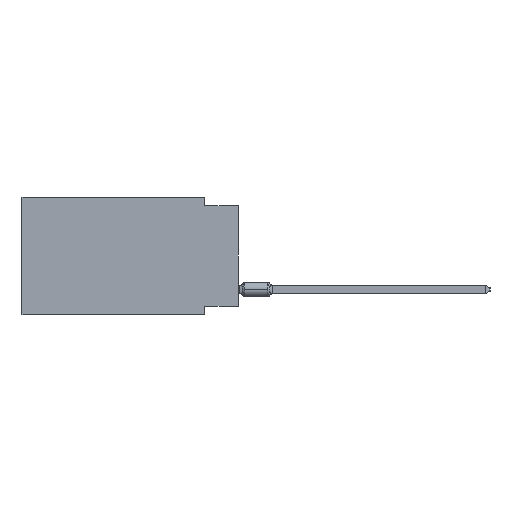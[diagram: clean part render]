
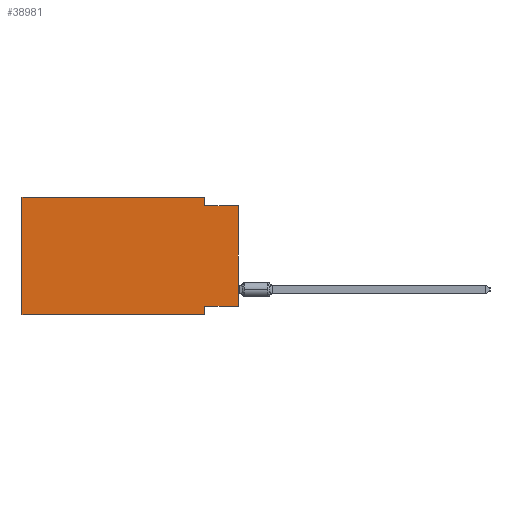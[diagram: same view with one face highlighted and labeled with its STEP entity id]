
A CAD part, left-side view. The second image highlights one B-rep face of the part: STEP entity #38981.
In plain terms, the highlighted planar face has unit normal (-1, 0, 0).
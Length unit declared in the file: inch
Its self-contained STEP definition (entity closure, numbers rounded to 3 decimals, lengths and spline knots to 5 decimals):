
#219 = VECTOR ( 'NONE', #7970, 39.37008 ) ;
#351 = DIRECTION ( 'NONE',  ( 0., 0., 1. ) ) ;
#927 = CARTESIAN_POINT ( 'NONE',  ( 0., 0.1, -0.325 ) ) ;
#3507 = ORIENTED_EDGE ( 'NONE', *, *, #48282, .F. ) ;
#4763 = CARTESIAN_POINT ( 'NONE',  ( 0., 0., -0.025 ) ) ;
#4801 = VERTEX_POINT ( 'NONE', #927 ) ;
#5118 = DIRECTION ( 'NONE',  ( 1., 0., 0. ) ) ;
#5246 = EDGE_CURVE ( 'NONE', #30728, #7656, #63425, .T. ) ;
#6955 = CARTESIAN_POINT ( 'NONE',  ( 0., 0.1, -0.35 ) ) ;
#7656 = VERTEX_POINT ( 'NONE', #24314 ) ;
#7919 = CARTESIAN_POINT ( 'NONE',  ( 0., 0., 0. ) ) ;
#7970 = DIRECTION ( 'NONE',  ( 0., -1., 0. ) ) ;
#8105 = EDGE_CURVE ( 'NONE', #7656, #64206, #9751, .T. ) ;
#8794 = DIRECTION ( 'NONE',  ( 0., -1., 0. ) ) ;
#9710 = LINE ( 'NONE', #46123, #57536 ) ;
#9751 = LINE ( 'NONE', #65556, #13404 ) ;
#10563 = VERTEX_POINT ( 'NONE', #36013 ) ;
#12307 = DIRECTION ( 'NONE',  ( 0., 0., -1. ) ) ;
#12536 = LINE ( 'NONE', #26581, #15799 ) ;
#13404 = VECTOR ( 'NONE', #19788, 39.37008 ) ;
#14592 = ORIENTED_EDGE ( 'NONE', *, *, #45447, .F. ) ;
#15783 = LINE ( 'NONE', #4763, #37073 ) ;
#15799 = VECTOR ( 'NONE', #57007, 39.37008 ) ;
#16535 = VERTEX_POINT ( 'NONE', #58576 ) ;
#16675 = LINE ( 'NONE', #6955, #18326 ) ;
#18326 = VECTOR ( 'NONE', #12307, 39.37008 ) ;
#19788 = DIRECTION ( 'NONE',  ( 0., 0., -1. ) ) ;
#20963 = ORIENTED_EDGE ( 'NONE', *, *, #8105, .F. ) ;
#22173 = VECTOR ( 'NONE', #58391, 39.37008 ) ;
#23159 = CARTESIAN_POINT ( 'NONE',  ( 0., 0.645, -0.35 ) ) ;
#24314 = CARTESIAN_POINT ( 'NONE',  ( 0., 0.1, 0. ) ) ;
#25510 = PLANE ( 'NONE',  #46611 ) ;
#25827 = FACE_OUTER_BOUND ( 'NONE', #31865, .T. ) ;
#25960 = CARTESIAN_POINT ( 'NONE',  ( 0., 0.1, -0.025 ) ) ;
#26371 = ORIENTED_EDGE ( 'NONE', *, *, #64893, .T. ) ;
#26581 = CARTESIAN_POINT ( 'NONE',  ( 0., 0., -0.325 ) ) ;
#28676 = EDGE_CURVE ( 'NONE', #16535, #61538, #53703, .T. ) ;
#30728 = VERTEX_POINT ( 'NONE', #41770 ) ;
#31443 = DIRECTION ( 'NONE',  ( 0., -1., 0. ) ) ;
#31865 = EDGE_LOOP ( 'NONE', ( #55086, #3507, #20963, #49716, #14592, #26371, #48968, #47297 ) ) ;
#32692 = CARTESIAN_POINT ( 'NONE',  ( 0., 0.645, 0. ) ) ;
#36013 = CARTESIAN_POINT ( 'NONE',  ( 0., 0.645, -0.35 ) ) ;
#37073 = VECTOR ( 'NONE', #31443, 39.37008 ) ;
#37854 = LINE ( 'NONE', #23159, #42801 ) ;
#38981 = ADVANCED_FACE ( 'NONE', ( #25827 ), #25510, .F. ) ;
#39543 = CARTESIAN_POINT ( 'NONE',  ( 0., 0.1, -0.35 ) ) ;
#40150 = VERTEX_POINT ( 'NONE', #39543 ) ;
#40848 = DIRECTION ( 'NONE',  ( 0., 0., -1. ) ) ;
#41770 = CARTESIAN_POINT ( 'NONE',  ( 0., 0.645, 0. ) ) ;
#42801 = VECTOR ( 'NONE', #8794, 39.37008 ) ;
#45447 = EDGE_CURVE ( 'NONE', #10563, #30728, #9710, .T. ) ;
#46123 = CARTESIAN_POINT ( 'NONE',  ( 0., 0.645, 0. ) ) ;
#46611 = AXIS2_PLACEMENT_3D ( 'NONE', #65942, #5118, #40848 ) ;
#47297 = ORIENTED_EDGE ( 'NONE', *, *, #61245, .F. ) ;
#48282 = EDGE_CURVE ( 'NONE', #64206, #61538, #15783, .T. ) ;
#48968 = ORIENTED_EDGE ( 'NONE', *, *, #65071, .F. ) ;
#49716 = ORIENTED_EDGE ( 'NONE', *, *, #5246, .F. ) ;
#53703 = LINE ( 'NONE', #7919, #22173 ) ;
#55086 = ORIENTED_EDGE ( 'NONE', *, *, #28676, .T. ) ;
#57007 = DIRECTION ( 'NONE',  ( 0., 1., 0. ) ) ;
#57536 = VECTOR ( 'NONE', #351, 39.37008 ) ;
#58391 = DIRECTION ( 'NONE',  ( 0., 0., 1. ) ) ;
#58576 = CARTESIAN_POINT ( 'NONE',  ( 0., 0., -0.325 ) ) ;
#61245 = EDGE_CURVE ( 'NONE', #16535, #4801, #12536, .T. ) ;
#61538 = VERTEX_POINT ( 'NONE', #65976 ) ;
#63425 = LINE ( 'NONE', #32692, #219 ) ;
#64206 = VERTEX_POINT ( 'NONE', #25960 ) ;
#64893 = EDGE_CURVE ( 'NONE', #10563, #40150, #37854, .T. ) ;
#65071 = EDGE_CURVE ( 'NONE', #4801, #40150, #16675, .T. ) ;
#65556 = CARTESIAN_POINT ( 'NONE',  ( 0., 0.1, 0. ) ) ;
#65942 = CARTESIAN_POINT ( 'NONE',  ( 0., 0.645, 0. ) ) ;
#65976 = CARTESIAN_POINT ( 'NONE',  ( 0., 0., -0.025 ) ) ;
